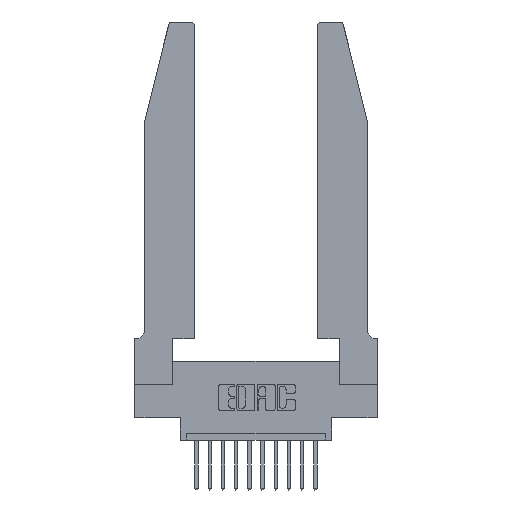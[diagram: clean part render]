
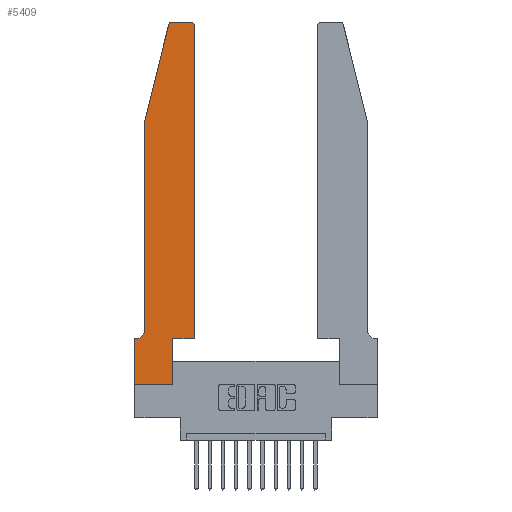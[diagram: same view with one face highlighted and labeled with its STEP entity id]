
A CAD part, top view. The second image highlights one B-rep face of the part: STEP entity #5409.
In plain terms, the highlighted planar face has unit normal (0, 0, 1).
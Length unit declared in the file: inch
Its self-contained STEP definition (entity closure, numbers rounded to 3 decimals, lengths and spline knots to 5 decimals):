
#14 = CARTESIAN_POINT ( 'NONE',  ( 0., 0.35, 0.37 ) ) ;
#531 = VERTEX_POINT ( 'NONE', #14 ) ;
#972 = CARTESIAN_POINT ( 'NONE',  ( 0.4505, 0.35, 0.37 ) ) ;
#981 = DIRECTION ( 'NONE',  ( -0.239, -0.971, 0. ) ) ;
#1390 = VECTOR ( 'NONE', #10314, 39.37008 ) ;
#1690 = DIRECTION ( 'NONE',  ( 0., 1., 0. ) ) ;
#1799 = AXIS2_PLACEMENT_3D ( 'NONE', #7768, #9082, #2616 ) ;
#2000 = VERTEX_POINT ( 'NONE', #3302 ) ;
#2048 = DIRECTION ( 'NONE',  ( 1., 0., 0. ) ) ;
#2199 = LINE ( 'NONE', #13989, #2804 ) ;
#2217 = LINE ( 'NONE', #9504, #9323 ) ;
#2404 = CIRCLE ( 'NONE', #11818, 0.07 ) ;
#2616 = DIRECTION ( 'NONE',  ( 1., 0., 0. ) ) ;
#2804 = VECTOR ( 'NONE', #4699, 39.37008 ) ;
#2842 = VERTEX_POINT ( 'NONE', #2980 ) ;
#2955 = ORIENTED_EDGE ( 'NONE', *, *, #8943, .T. ) ;
#2971 = DIRECTION ( 'NONE',  ( 0., -1., 0. ) ) ;
#2979 = CARTESIAN_POINT ( 'NONE',  ( 0., 0.35, 0.37 ) ) ;
#2980 = CARTESIAN_POINT ( 'NONE',  ( 0.2865, 0.35, 0.37 ) ) ;
#3016 = VECTOR ( 'NONE', #981, 39.37008 ) ;
#3055 = AXIS2_PLACEMENT_3D ( 'NONE', #5780, #3214, #13610 ) ;
#3214 = DIRECTION ( 'NONE',  ( 0., 0., 1. ) ) ;
#3259 = CIRCLE ( 'NONE', #3055, 0.03 ) ;
#3302 = CARTESIAN_POINT ( 'NONE',  ( 0.4205, 2.75, 0.37 ) ) ;
#3796 = EDGE_CURVE ( 'NONE', #4007, #13182, #5905, .T. ) ;
#3807 = DIRECTION ( 'NONE',  ( 0., 1., 0. ) ) ;
#3924 = EDGE_CURVE ( 'NONE', #2842, #16478, #8729, .T. ) ;
#4007 = VERTEX_POINT ( 'NONE', #5724 ) ;
#4080 = CARTESIAN_POINT ( 'NONE',  ( 0.0055, 0.42, 0.37 ) ) ;
#4106 = ORIENTED_EDGE ( 'NONE', *, *, #14181, .T. ) ;
#4346 = CARTESIAN_POINT ( 'NONE',  ( 0., 0., 0.37 ) ) ;
#4414 = FACE_OUTER_BOUND ( 'NONE', #7570, .T. ) ;
#4434 = CARTESIAN_POINT ( 'NONE',  ( 0.0755, 0.35, 0.37 ) ) ;
#4449 = EDGE_CURVE ( 'NONE', #2000, #4007, #2199, .T. ) ;
#4550 = CARTESIAN_POINT ( 'NONE',  ( 0.0755, 2., 0.37 ) ) ;
#4699 = DIRECTION ( 'NONE',  ( -1., 0., 0. ) ) ;
#4827 = LINE ( 'NONE', #4346, #15541 ) ;
#5013 = LINE ( 'NONE', #6301, #14131 ) ;
#5021 = LINE ( 'NONE', #16278, #11531 ) ;
#5409 = ADVANCED_FACE ( 'NONE', ( #4414 ), #9120, .T. ) ;
#5437 = EDGE_CURVE ( 'NONE', #14107, #12720, #5021, .T. ) ;
#5685 = ORIENTED_EDGE ( 'NONE', *, *, #4449, .T. ) ;
#5724 = CARTESIAN_POINT ( 'NONE',  ( 0.284, 2.75, 0.37 ) ) ;
#5780 = CARTESIAN_POINT ( 'NONE',  ( 0.4205, 2.72, 0.37 ) ) ;
#5905 = CIRCLE ( 'NONE', #1799, 0.03 ) ;
#6301 = CARTESIAN_POINT ( 'NONE',  ( 0.2865, 0.35, 0.37 ) ) ;
#6864 = VERTEX_POINT ( 'NONE', #9299 ) ;
#7118 = ORIENTED_EDGE ( 'NONE', *, *, #5437, .T. ) ;
#7330 = ORIENTED_EDGE ( 'NONE', *, *, #3796, .T. ) ;
#7570 = EDGE_LOOP ( 'NONE', ( #5685, #7330, #2955, #7118, #8846, #4106, #11330, #13683, #12546, #9160, #11718, #12756 ) ) ;
#7768 = CARTESIAN_POINT ( 'NONE',  ( 0.284, 2.72, 0.37 ) ) ;
#7932 = EDGE_CURVE ( 'NONE', #11238, #2000, #3259, .T. ) ;
#8112 = LINE ( 'NONE', #12674, #3016 ) ;
#8125 = CARTESIAN_POINT ( 'NONE',  ( 0.0755, 0.42, 0.37 ) ) ;
#8314 = VECTOR ( 'NONE', #11255, 39.37008 ) ;
#8553 = EDGE_CURVE ( 'NONE', #16478, #11238, #2217, .T. ) ;
#8729 = LINE ( 'NONE', #8997, #1390 ) ;
#8846 = ORIENTED_EDGE ( 'NONE', *, *, #9515, .T. ) ;
#8853 = CARTESIAN_POINT ( 'NONE',  ( 0.4505, 2.72, 0.37 ) ) ;
#8943 = EDGE_CURVE ( 'NONE', #13182, #14107, #8112, .T. ) ;
#8997 = CARTESIAN_POINT ( 'NONE',  ( 0.4505, 0.35, 0.37 ) ) ;
#9073 = CARTESIAN_POINT ( 'NONE',  ( 0.2865, 0., 0.37 ) ) ;
#9082 = DIRECTION ( 'NONE',  ( 0., 0., 1. ) ) ;
#9120 = PLANE ( 'NONE',  #12294 ) ;
#9160 = ORIENTED_EDGE ( 'NONE', *, *, #3924, .T. ) ;
#9299 = CARTESIAN_POINT ( 'NONE',  ( 0., 0., 0.37 ) ) ;
#9323 = VECTOR ( 'NONE', #1690, 39.37008 ) ;
#9504 = CARTESIAN_POINT ( 'NONE',  ( 0.4505, 0.35, 0.37 ) ) ;
#9515 = EDGE_CURVE ( 'NONE', #12720, #12663, #2404, .T. ) ;
#10216 = EDGE_CURVE ( 'NONE', #531, #6864, #4827, .T. ) ;
#10314 = DIRECTION ( 'NONE',  ( 1., 0., 0. ) ) ;
#10511 = CARTESIAN_POINT ( 'NONE',  ( 0.0055, 0.35, 0.37 ) ) ;
#10610 = DIRECTION ( 'NONE',  ( -1., 0., 0. ) ) ;
#10890 = DIRECTION ( 'NONE',  ( 0., 0., 1. ) ) ;
#11238 = VERTEX_POINT ( 'NONE', #8853 ) ;
#11255 = DIRECTION ( 'NONE',  ( -1., 0., 0. ) ) ;
#11330 = ORIENTED_EDGE ( 'NONE', *, *, #10216, .T. ) ;
#11348 = VECTOR ( 'NONE', #2048, 39.37008 ) ;
#11531 = VECTOR ( 'NONE', #15110, 39.37008 ) ;
#11718 = ORIENTED_EDGE ( 'NONE', *, *, #8553, .T. ) ;
#11818 = AXIS2_PLACEMENT_3D ( 'NONE', #4080, #13209, #10610 ) ;
#12294 = AXIS2_PLACEMENT_3D ( 'NONE', #2979, #10890, #13043 ) ;
#12546 = ORIENTED_EDGE ( 'NONE', *, *, #16592, .T. ) ;
#12663 = VERTEX_POINT ( 'NONE', #10511 ) ;
#12674 = CARTESIAN_POINT ( 'NONE',  ( 0.0755, 2., 0.37 ) ) ;
#12720 = VERTEX_POINT ( 'NONE', #8125 ) ;
#12744 = CARTESIAN_POINT ( 'NONE',  ( 0.25487, 2.72718, 0.37 ) ) ;
#12756 = ORIENTED_EDGE ( 'NONE', *, *, #7932, .T. ) ;
#13043 = DIRECTION ( 'NONE',  ( 1., 0., 0. ) ) ;
#13182 = VERTEX_POINT ( 'NONE', #12744 ) ;
#13209 = DIRECTION ( 'NONE',  ( 0., 0., -1. ) ) ;
#13353 = LINE ( 'NONE', #13591, #11348 ) ;
#13591 = CARTESIAN_POINT ( 'NONE',  ( 0., 0., 0.37 ) ) ;
#13610 = DIRECTION ( 'NONE',  ( 1., 0., 0. ) ) ;
#13683 = ORIENTED_EDGE ( 'NONE', *, *, #15418, .T. ) ;
#13989 = CARTESIAN_POINT ( 'NONE',  ( 0.2605, 2.75, 0.37 ) ) ;
#14107 = VERTEX_POINT ( 'NONE', #4550 ) ;
#14131 = VECTOR ( 'NONE', #3807, 39.37008 ) ;
#14181 = EDGE_CURVE ( 'NONE', #12663, #531, #14193, .T. ) ;
#14193 = LINE ( 'NONE', #4434, #8314 ) ;
#14431 = VERTEX_POINT ( 'NONE', #9073 ) ;
#15110 = DIRECTION ( 'NONE',  ( 0., -1., 0. ) ) ;
#15418 = EDGE_CURVE ( 'NONE', #6864, #14431, #13353, .T. ) ;
#15541 = VECTOR ( 'NONE', #2971, 39.37008 ) ;
#16278 = CARTESIAN_POINT ( 'NONE',  ( 0.0755, 2., 0.37 ) ) ;
#16478 = VERTEX_POINT ( 'NONE', #972 ) ;
#16592 = EDGE_CURVE ( 'NONE', #14431, #2842, #5013, .T. ) ;
